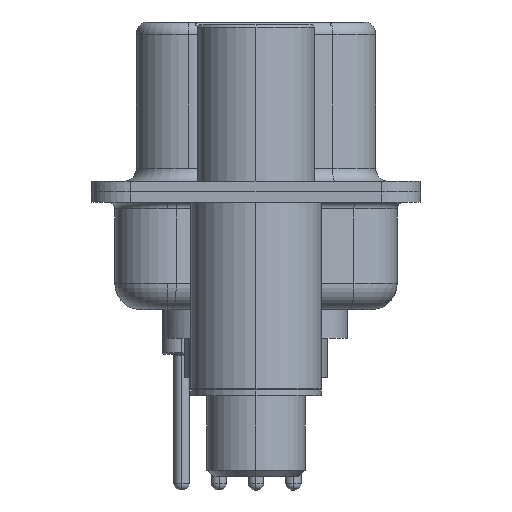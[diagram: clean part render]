
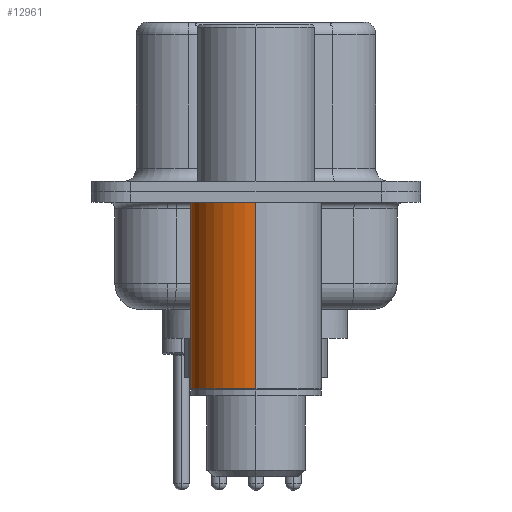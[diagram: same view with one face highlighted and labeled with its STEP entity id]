
A CAD part, left-side view. The second image highlights one B-rep face of the part: STEP entity #12961.
In plain terms, the highlighted cylindrical face has radius 2.5 mm (diameter 5 mm), a partial arc.
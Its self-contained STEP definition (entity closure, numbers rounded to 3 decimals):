
#890 = VERTEX_POINT ( 'NONE', #18925 ) ;
#1526 = VERTEX_POINT ( 'NONE', #14524 ) ;
#1640 = ORIENTED_EDGE ( 'NONE', *, *, #4227, .F. ) ;
#2334 = CARTESIAN_POINT ( 'NONE',  ( 0., 0., -0.4 ) ) ;
#2409 = VECTOR ( 'NONE', #19947, 1000. ) ;
#2850 = CARTESIAN_POINT ( 'NONE',  ( 2.5, 0., -0.4 ) ) ;
#3047 = ORIENTED_EDGE ( 'NONE', *, *, #13563, .T. ) ;
#3052 = FACE_OUTER_BOUND ( 'NONE', #16309, .T. ) ;
#3708 = DIRECTION ( 'NONE',  ( 1., 0., 0. ) ) ;
#3969 = DIRECTION ( 'NONE',  ( 0., 0., 1. ) ) ;
#4087 = DIRECTION ( 'NONE',  ( 1., 0., 0. ) ) ;
#4227 = EDGE_CURVE ( 'NONE', #5936, #20065, #17029, .T. ) ;
#5936 = VERTEX_POINT ( 'NONE', #21471 ) ;
#6459 = LINE ( 'NONE', #6506, #2409 ) ;
#6506 = CARTESIAN_POINT ( 'NONE',  ( -2.5, 0., 0.581 ) ) ;
#7214 = AXIS2_PLACEMENT_3D ( 'NONE', #14110, #3969, #15843 ) ;
#11057 = DIRECTION ( 'NONE',  ( 0., 0., 1. ) ) ;
#12076 = EDGE_CURVE ( 'NONE', #20065, #1526, #19852, .T. ) ;
#12229 = CARTESIAN_POINT ( 'NONE',  ( 0., 0., 0.581 ) ) ;
#12589 = ORIENTED_EDGE ( 'NONE', *, *, #15898, .T. ) ;
#12961 = ADVANCED_FACE ( 'NONE', ( #3052 ), #16103, .T. ) ;
#13079 = AXIS2_PLACEMENT_3D ( 'NONE', #2334, #14241, #4087 ) ;
#13563 = EDGE_CURVE ( 'NONE', #5936, #890, #20079, .T. ) ;
#14110 = CARTESIAN_POINT ( 'NONE',  ( 0., 0., -7.525 ) ) ;
#14241 = DIRECTION ( 'NONE',  ( 0., 0., 1. ) ) ;
#14524 = CARTESIAN_POINT ( 'NONE',  ( -2.5, 0., -0.4 ) ) ;
#15557 = DIRECTION ( 'NONE',  ( 0., 0., 1. ) ) ;
#15843 = DIRECTION ( 'NONE',  ( 1., 0., 0. ) ) ;
#15898 = EDGE_CURVE ( 'NONE', #890, #1526, #6459, .T. ) ;
#16103 = CYLINDRICAL_SURFACE ( 'NONE', #22167, 2.5 ) ;
#16309 = EDGE_LOOP ( 'NONE', ( #3047, #12589, #17634, #1640 ) ) ;
#17029 = LINE ( 'NONE', #20535, #21587 ) ;
#17634 = ORIENTED_EDGE ( 'NONE', *, *, #12076, .F. ) ;
#18925 = CARTESIAN_POINT ( 'NONE',  ( -2.5, 0., -7.525 ) ) ;
#19852 = CIRCLE ( 'NONE', #13079, 2.5 ) ;
#19947 = DIRECTION ( 'NONE',  ( 0., 0., 1. ) ) ;
#20065 = VERTEX_POINT ( 'NONE', #2850 ) ;
#20079 = CIRCLE ( 'NONE', #7214, 2.5 ) ;
#20535 = CARTESIAN_POINT ( 'NONE',  ( 2.5, 0., 0.581 ) ) ;
#21471 = CARTESIAN_POINT ( 'NONE',  ( 2.5, 0., -7.525 ) ) ;
#21587 = VECTOR ( 'NONE', #11057, 1000. ) ;
#22167 = AXIS2_PLACEMENT_3D ( 'NONE', #12229, #15557, #3708 ) ;
